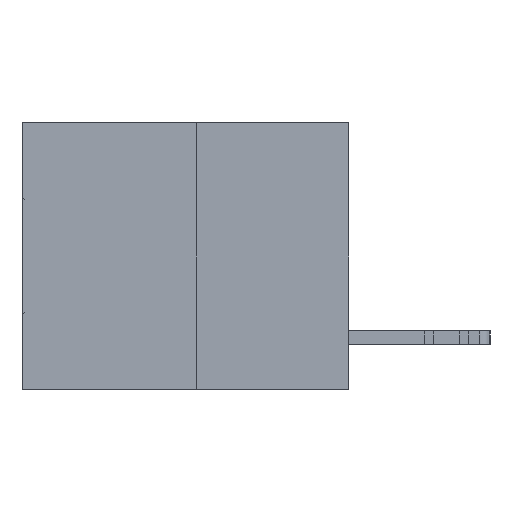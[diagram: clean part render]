
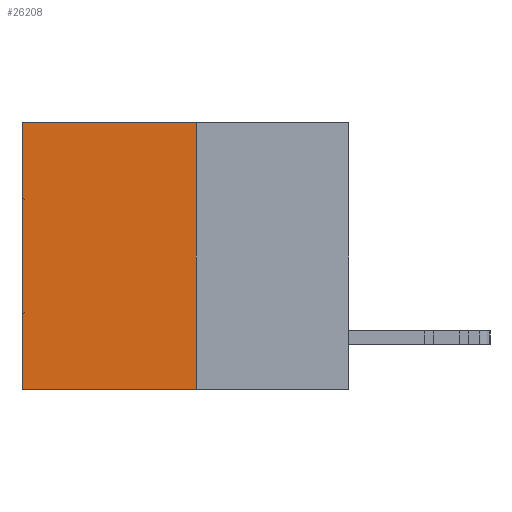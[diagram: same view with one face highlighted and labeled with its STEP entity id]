
A CAD part, left-side view. The second image highlights one B-rep face of the part: STEP entity #26208.
In plain terms, the highlighted planar face has unit normal (-1, 0, 0).
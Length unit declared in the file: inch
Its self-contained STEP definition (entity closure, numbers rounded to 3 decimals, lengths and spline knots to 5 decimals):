
#1319 = DIRECTION ( 'NONE',  ( 0., 0., -1. ) ) ;
#1382 = CARTESIAN_POINT ( 'NONE',  ( 0.3165, 0.28, -0.49 ) ) ;
#1770 = EDGE_CURVE ( 'NONE', #10599, #14717, #16750, .T. ) ;
#2422 = EDGE_CURVE ( 'NONE', #10599, #29831, #2767, .T. ) ;
#2767 = LINE ( 'NONE', #18330, #12025 ) ;
#3093 = DIRECTION ( 'NONE',  ( 0., 1., 0. ) ) ;
#3547 = ORIENTED_EDGE ( 'NONE', *, *, #2422, .T. ) ;
#4901 = LINE ( 'NONE', #31886, #12261 ) ;
#5335 = CARTESIAN_POINT ( 'NONE',  ( 0.3165, 0.28, -0.49 ) ) ;
#8482 = EDGE_CURVE ( 'NONE', #29831, #9926, #4901, .T. ) ;
#8588 = DIRECTION ( 'NONE',  ( 1., 0., 0. ) ) ;
#9697 = LINE ( 'NONE', #5335, #15922 ) ;
#9926 = VERTEX_POINT ( 'NONE', #23923 ) ;
#10599 = VERTEX_POINT ( 'NONE', #15068 ) ;
#11541 = EDGE_CURVE ( 'NONE', #14717, #9926, #9697, .T. ) ;
#12025 = VECTOR ( 'NONE', #28247, 39.37008 ) ;
#12261 = VECTOR ( 'NONE', #19524, 39.37008 ) ;
#13555 = CARTESIAN_POINT ( 'NONE',  ( 0.3165, 0.28, -0.49 ) ) ;
#13934 = PLANE ( 'NONE',  #18630 ) ;
#14717 = VERTEX_POINT ( 'NONE', #13555 ) ;
#15068 = CARTESIAN_POINT ( 'NONE',  ( 0.3165, 0.28, 0. ) ) ;
#15635 = VECTOR ( 'NONE', #1319, 39.37008 ) ;
#15922 = VECTOR ( 'NONE', #3093, 39.37008 ) ;
#15975 = DIRECTION ( 'NONE',  ( 0., 0., -1. ) ) ;
#16750 = LINE ( 'NONE', #18464, #15635 ) ;
#17460 = CARTESIAN_POINT ( 'NONE',  ( 0.3165, 0.6, 0. ) ) ;
#18264 = ORIENTED_EDGE ( 'NONE', *, *, #1770, .F. ) ;
#18330 = CARTESIAN_POINT ( 'NONE',  ( 0.3165, 0.28, 0. ) ) ;
#18464 = CARTESIAN_POINT ( 'NONE',  ( 0.3165, 0.28, -0.49 ) ) ;
#18630 = AXIS2_PLACEMENT_3D ( 'NONE', #1382, #8588, #15975 ) ;
#19524 = DIRECTION ( 'NONE',  ( 0., 0., -1. ) ) ;
#23835 = EDGE_LOOP ( 'NONE', ( #29148, #28579, #18264, #3547 ) ) ;
#23923 = CARTESIAN_POINT ( 'NONE',  ( 0.3165, 0.6, -0.49 ) ) ;
#26208 = ADVANCED_FACE ( 'NONE', ( #27653 ), #13934, .F. ) ;
#27653 = FACE_OUTER_BOUND ( 'NONE', #23835, .T. ) ;
#28247 = DIRECTION ( 'NONE',  ( 0., 1., 0. ) ) ;
#28579 = ORIENTED_EDGE ( 'NONE', *, *, #11541, .F. ) ;
#29148 = ORIENTED_EDGE ( 'NONE', *, *, #8482, .T. ) ;
#29831 = VERTEX_POINT ( 'NONE', #17460 ) ;
#31886 = CARTESIAN_POINT ( 'NONE',  ( 0.3165, 0.6, -0.49 ) ) ;
